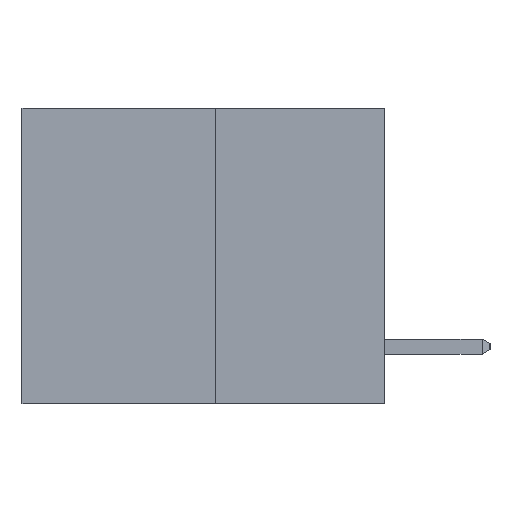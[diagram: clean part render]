
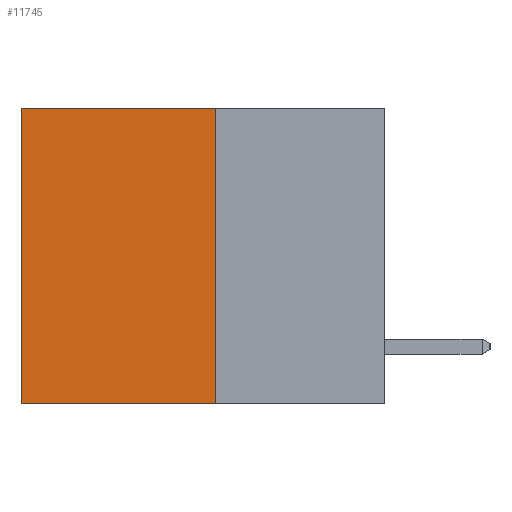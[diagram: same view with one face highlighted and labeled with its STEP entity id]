
A CAD part, left-side view. The second image highlights one B-rep face of the part: STEP entity #11745.
In plain terms, the highlighted planar face has unit normal (-1, 0, 0).
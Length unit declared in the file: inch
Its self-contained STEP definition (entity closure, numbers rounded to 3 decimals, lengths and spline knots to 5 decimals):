
#1330 = DIRECTION ( 'NONE',  ( 0., 1., 0. ) ) ;
#3245 = LINE ( 'NONE', #11137, #21184 ) ;
#3464 = VERTEX_POINT ( 'NONE', #17076 ) ;
#4128 = CARTESIAN_POINT ( 'NONE',  ( 0.3165, 0.6, 0. ) ) ;
#4249 = DIRECTION ( 'NONE',  ( 1., 0., 0. ) ) ;
#4396 = CARTESIAN_POINT ( 'NONE',  ( 0.3165, 0.28, -0.49 ) ) ;
#5692 = CARTESIAN_POINT ( 'NONE',  ( 0.3165, 0.28, 0. ) ) ;
#5924 = DIRECTION ( 'NONE',  ( 0., 1., 0. ) ) ;
#6060 = VECTOR ( 'NONE', #1330, 39.37008 ) ;
#7107 = VERTEX_POINT ( 'NONE', #22169 ) ;
#7592 = DIRECTION ( 'NONE',  ( 0., 0., -1. ) ) ;
#7668 = CARTESIAN_POINT ( 'NONE',  ( 0.3165, 0.6, -0.49 ) ) ;
#8211 = EDGE_LOOP ( 'NONE', ( #21142, #18843, #14047, #13164 ) ) ;
#8269 = FACE_OUTER_BOUND ( 'NONE', #8211, .T. ) ;
#9132 = EDGE_CURVE ( 'NONE', #11903, #3464, #22104, .T. ) ;
#9330 = DIRECTION ( 'NONE',  ( 0., 0., -1. ) ) ;
#11137 = CARTESIAN_POINT ( 'NONE',  ( 0.3165, 0.28, -0.49 ) ) ;
#11745 = ADVANCED_FACE ( 'NONE', ( #8269 ), #18177, .F. ) ;
#11903 = VERTEX_POINT ( 'NONE', #4128 ) ;
#12033 = VERTEX_POINT ( 'NONE', #12391 ) ;
#12391 = CARTESIAN_POINT ( 'NONE',  ( 0.3165, 0.28, -0.49 ) ) ;
#12593 = AXIS2_PLACEMENT_3D ( 'NONE', #4396, #4249, #16621 ) ;
#12993 = LINE ( 'NONE', #5692, #6060 ) ;
#13164 = ORIENTED_EDGE ( 'NONE', *, *, #21881, .T. ) ;
#13177 = CARTESIAN_POINT ( 'NONE',  ( 0.3165, 0.28, -0.49 ) ) ;
#14047 = ORIENTED_EDGE ( 'NONE', *, *, #15525, .F. ) ;
#15525 = EDGE_CURVE ( 'NONE', #7107, #12033, #3245, .T. ) ;
#16064 = LINE ( 'NONE', #13177, #21245 ) ;
#16621 = DIRECTION ( 'NONE',  ( 0., 0., -1. ) ) ;
#17076 = CARTESIAN_POINT ( 'NONE',  ( 0.3165, 0.6, -0.49 ) ) ;
#17493 = VECTOR ( 'NONE', #7592, 39.37008 ) ;
#18177 = PLANE ( 'NONE',  #12593 ) ;
#18843 = ORIENTED_EDGE ( 'NONE', *, *, #20965, .F. ) ;
#20965 = EDGE_CURVE ( 'NONE', #12033, #3464, #16064, .T. ) ;
#21142 = ORIENTED_EDGE ( 'NONE', *, *, #9132, .T. ) ;
#21184 = VECTOR ( 'NONE', #9330, 39.37008 ) ;
#21245 = VECTOR ( 'NONE', #5924, 39.37008 ) ;
#21881 = EDGE_CURVE ( 'NONE', #7107, #11903, #12993, .T. ) ;
#22104 = LINE ( 'NONE', #7668, #17493 ) ;
#22169 = CARTESIAN_POINT ( 'NONE',  ( 0.3165, 0.28, 0. ) ) ;
